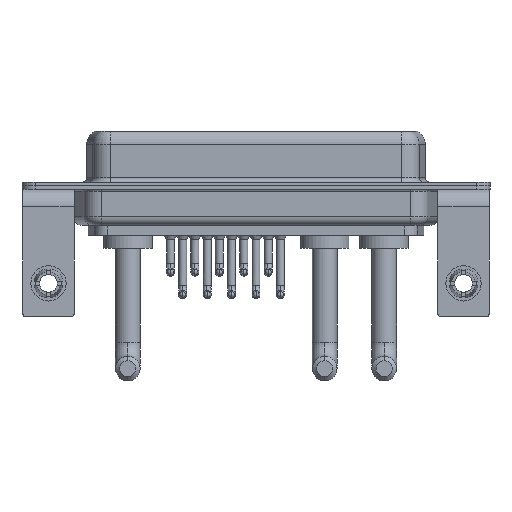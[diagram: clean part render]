
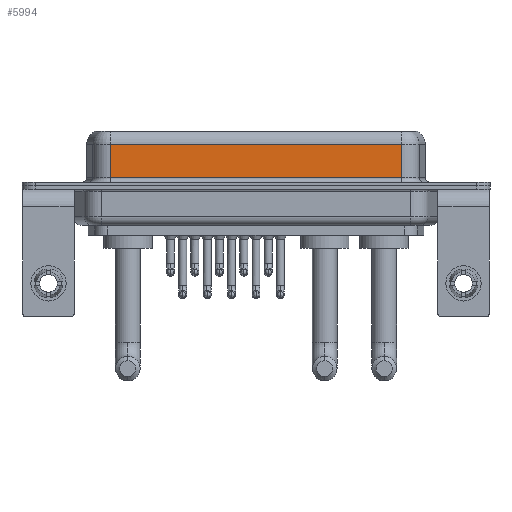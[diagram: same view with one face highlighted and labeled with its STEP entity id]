
A CAD part, front view. The second image highlights one B-rep face of the part: STEP entity #5994.
In plain terms, the highlighted planar face has unit normal (0, -1, 0).
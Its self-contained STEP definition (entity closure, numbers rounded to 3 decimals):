
#304 = DIRECTION ( 'NONE',  ( 0., 1., 0. ) ) ;
#732 = CARTESIAN_POINT ( 'NONE',  ( 40.037, -3.95, 6.4 ) ) ;
#879 = VECTOR ( 'NONE', #9377, 1000. ) ;
#1070 = DIRECTION ( 'NONE',  ( 0., 0., -1. ) ) ;
#1288 = ORIENTED_EDGE ( 'NONE', *, *, #20675, .T. ) ;
#1972 = EDGE_CURVE ( 'NONE', #18295, #2584, #19302, .T. ) ;
#2100 = CARTESIAN_POINT ( 'NONE',  ( 7.013, -3.95, 0.9 ) ) ;
#2584 = VERTEX_POINT ( 'NONE', #20318 ) ;
#2932 = CARTESIAN_POINT ( 'NONE',  ( 40.037, -3.95, 6.4 ) ) ;
#3426 = VERTEX_POINT ( 'NONE', #9761 ) ;
#3786 = FACE_OUTER_BOUND ( 'NONE', #6080, .T. ) ;
#3856 = LINE ( 'NONE', #10367, #12704 ) ;
#4376 = LINE ( 'NONE', #15976, #879 ) ;
#4915 = VERTEX_POINT ( 'NONE', #2100 ) ;
#5994 = ADVANCED_FACE ( 'NONE', ( #3786 ), #15580, .F. ) ;
#6080 = EDGE_LOOP ( 'NONE', ( #8656, #1288, #11041, #12779 ) ) ;
#6357 = EDGE_CURVE ( 'NONE', #3426, #4915, #3856, .T. ) ;
#6922 = DIRECTION ( 'NONE',  ( 0., 0., 1. ) ) ;
#8656 = ORIENTED_EDGE ( 'NONE', *, *, #1972, .F. ) ;
#9377 = DIRECTION ( 'NONE',  ( 1., 0., 0. ) ) ;
#9761 = CARTESIAN_POINT ( 'NONE',  ( 7.013, -3.95, 4.65 ) ) ;
#9949 = CARTESIAN_POINT ( 'NONE',  ( 40.037, -3.95, 4.65 ) ) ;
#10059 = LINE ( 'NONE', #9949, #19710 ) ;
#10367 = CARTESIAN_POINT ( 'NONE',  ( 7.013, -3.95, 6.4 ) ) ;
#11041 = ORIENTED_EDGE ( 'NONE', *, *, #6357, .T. ) ;
#11670 = DIRECTION ( 'NONE',  ( -1., 0., 0. ) ) ;
#12131 = EDGE_CURVE ( 'NONE', #4915, #2584, #4376, .T. ) ;
#12704 = VECTOR ( 'NONE', #18619, 1000. ) ;
#12779 = ORIENTED_EDGE ( 'NONE', *, *, #12131, .T. ) ;
#14952 = CARTESIAN_POINT ( 'NONE',  ( 40.037, -3.95, 4.65 ) ) ;
#15462 = AXIS2_PLACEMENT_3D ( 'NONE', #732, #304, #6922 ) ;
#15580 = PLANE ( 'NONE',  #15462 ) ;
#15976 = CARTESIAN_POINT ( 'NONE',  ( 40.037, -3.95, 0.9 ) ) ;
#18295 = VERTEX_POINT ( 'NONE', #14952 ) ;
#18619 = DIRECTION ( 'NONE',  ( 0., 0., -1. ) ) ;
#19302 = LINE ( 'NONE', #2932, #20618 ) ;
#19710 = VECTOR ( 'NONE', #11670, 1000. ) ;
#20318 = CARTESIAN_POINT ( 'NONE',  ( 40.037, -3.95, 0.9 ) ) ;
#20618 = VECTOR ( 'NONE', #1070, 1000. ) ;
#20675 = EDGE_CURVE ( 'NONE', #18295, #3426, #10059, .T. ) ;
